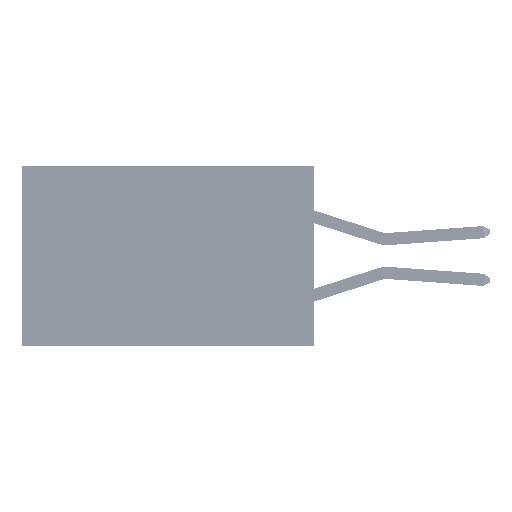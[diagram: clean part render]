
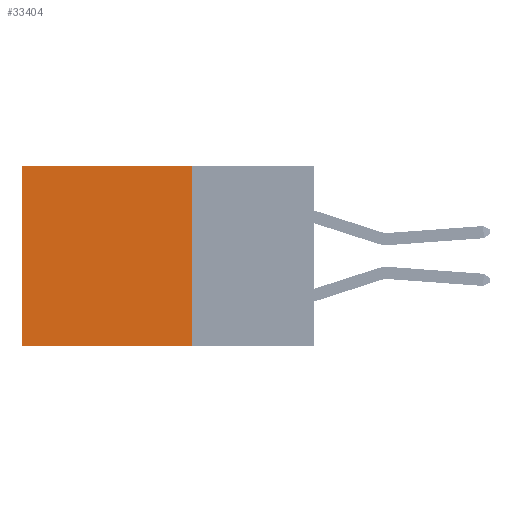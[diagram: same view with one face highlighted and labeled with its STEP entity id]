
A CAD part, left-side view. The second image highlights one B-rep face of the part: STEP entity #33404.
In plain terms, the highlighted planar face has unit normal (-1, 0, 0).
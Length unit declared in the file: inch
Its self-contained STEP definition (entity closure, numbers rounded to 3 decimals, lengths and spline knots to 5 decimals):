
#605 = EDGE_CURVE ( 'NONE', #10526, #6525, #15811, .T. ) ;
#1987 = CARTESIAN_POINT ( 'NONE',  ( 0.2875, 0.25, -0.37 ) ) ;
#2193 = VECTOR ( 'NONE', #32336, 39.37008 ) ;
#3267 = EDGE_CURVE ( 'NONE', #6525, #25425, #36415, .T. ) ;
#6525 = VERTEX_POINT ( 'NONE', #1987 ) ;
#7198 = CARTESIAN_POINT ( 'NONE',  ( 0.2875, 0.25, 0. ) ) ;
#8655 = DIRECTION ( 'NONE',  ( 0., 0., -1. ) ) ;
#9154 = CARTESIAN_POINT ( 'NONE',  ( 0.2875, 0.25, 0. ) ) ;
#9621 = DIRECTION ( 'NONE',  ( 1., 0., 0. ) ) ;
#9951 = ORIENTED_EDGE ( 'NONE', *, *, #45813, .T. ) ;
#10526 = VERTEX_POINT ( 'NONE', #7198 ) ;
#15811 = LINE ( 'NONE', #41322, #23660 ) ;
#17772 = CARTESIAN_POINT ( 'NONE',  ( 0.2875, 0.6, 0. ) ) ;
#17910 = ORIENTED_EDGE ( 'NONE', *, *, #44179, .T. ) ;
#19228 = CARTESIAN_POINT ( 'NONE',  ( 0.2875, 0.6, -0.37 ) ) ;
#19627 = FACE_OUTER_BOUND ( 'NONE', #30075, .T. ) ;
#20932 = CARTESIAN_POINT ( 'NONE',  ( 0.2875, 0.6, 0. ) ) ;
#21117 = LINE ( 'NONE', #17772, #2193 ) ;
#22332 = CARTESIAN_POINT ( 'NONE',  ( 0.2875, 0.25, 0. ) ) ;
#23453 = DIRECTION ( 'NONE',  ( 0., 0., -1. ) ) ;
#23660 = VECTOR ( 'NONE', #8655, 39.37008 ) ;
#25425 = VERTEX_POINT ( 'NONE', #19228 ) ;
#28609 = VERTEX_POINT ( 'NONE', #20932 ) ;
#29357 = ORIENTED_EDGE ( 'NONE', *, *, #3267, .F. ) ;
#30075 = EDGE_LOOP ( 'NONE', ( #17910, #29357, #30873, #9951 ) ) ;
#30873 = ORIENTED_EDGE ( 'NONE', *, *, #605, .F. ) ;
#32336 = DIRECTION ( 'NONE',  ( 0., 0., -1. ) ) ;
#32380 = DIRECTION ( 'NONE',  ( 0., 1., 0. ) ) ;
#33071 = LINE ( 'NONE', #22332, #46978 ) ;
#33404 = ADVANCED_FACE ( 'NONE', ( #19627 ), #34197, .F. ) ;
#34197 = PLANE ( 'NONE',  #35810 ) ;
#35810 = AXIS2_PLACEMENT_3D ( 'NONE', #9154, #9621, #23453 ) ;
#36415 = LINE ( 'NONE', #40461, #43275 ) ;
#36883 = DIRECTION ( 'NONE',  ( 0., 1., 0. ) ) ;
#40461 = CARTESIAN_POINT ( 'NONE',  ( 0.2875, 0.25, -0.37 ) ) ;
#41322 = CARTESIAN_POINT ( 'NONE',  ( 0.2875, 0.25, 0. ) ) ;
#43275 = VECTOR ( 'NONE', #32380, 39.37008 ) ;
#44179 = EDGE_CURVE ( 'NONE', #28609, #25425, #21117, .T. ) ;
#45813 = EDGE_CURVE ( 'NONE', #10526, #28609, #33071, .T. ) ;
#46978 = VECTOR ( 'NONE', #36883, 39.37008 ) ;
